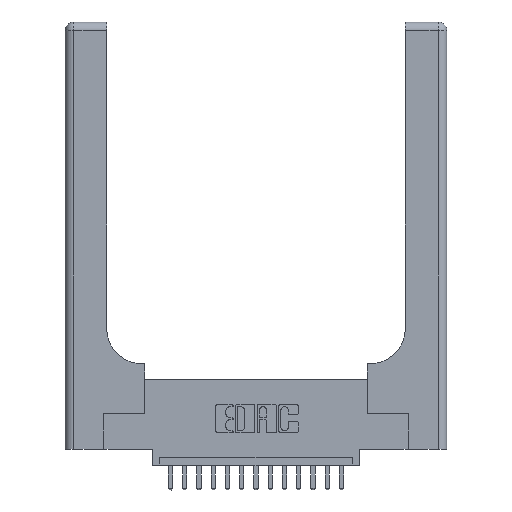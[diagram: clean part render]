
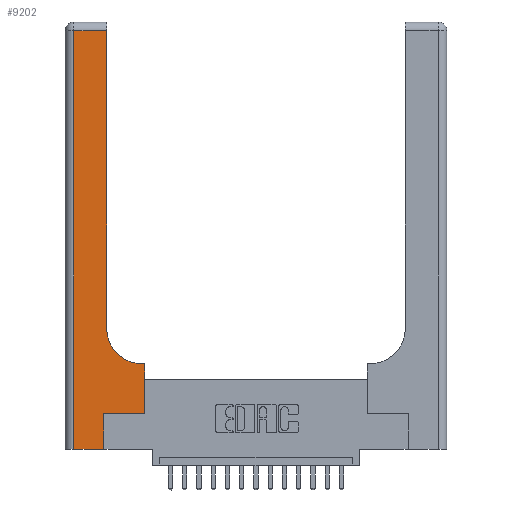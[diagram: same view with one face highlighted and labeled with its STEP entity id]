
A CAD part, top view. The second image highlights one B-rep face of the part: STEP entity #9202.
In plain terms, the highlighted planar face has unit normal (0, 0, 1).
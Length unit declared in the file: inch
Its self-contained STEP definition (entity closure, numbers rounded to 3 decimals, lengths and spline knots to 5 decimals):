
#174 = ORIENTED_EDGE ( 'NONE', *, *, #14792, .T. ) ;
#429 = AXIS2_PLACEMENT_3D ( 'NONE', #8814, #2917, #16340 ) ;
#547 = LINE ( 'NONE', #15109, #12341 ) ;
#780 = LINE ( 'NONE', #13860, #5628 ) ;
#890 = DIRECTION ( 'NONE',  ( -1., 0., 0. ) ) ;
#905 = VECTOR ( 'NONE', #5362, 39.37008 ) ;
#1137 = ORIENTED_EDGE ( 'NONE', *, *, #15764, .T. ) ;
#1366 = CARTESIAN_POINT ( 'NONE',  ( 0.5415, 0.6, 0.37 ) ) ;
#1576 = AXIS2_PLACEMENT_3D ( 'NONE', #3415, #16846, #8022 ) ;
#1577 = VERTEX_POINT ( 'NONE', #15545 ) ;
#1743 = ORIENTED_EDGE ( 'NONE', *, *, #8934, .T. ) ;
#1853 = DIRECTION ( 'NONE',  ( 0., -1., 0. ) ) ;
#2070 = CARTESIAN_POINT ( 'NONE',  ( 0.5585, 0.25, 0.37 ) ) ;
#2392 = ORIENTED_EDGE ( 'NONE', *, *, #12185, .T. ) ;
#2446 = VECTOR ( 'NONE', #13163, 39.37008 ) ;
#2524 = EDGE_CURVE ( 'NONE', #10962, #1577, #6870, .T. ) ;
#2917 = DIRECTION ( 'NONE',  ( 0., 0., -1. ) ) ;
#3000 = LINE ( 'NONE', #2070, #18255 ) ;
#3244 = VERTEX_POINT ( 'NONE', #11967 ) ;
#3305 = DIRECTION ( 'NONE',  ( 0., 1., 0. ) ) ;
#3332 = LINE ( 'NONE', #14197, #3804 ) ;
#3349 = LINE ( 'NONE', #17883, #9839 ) ;
#3415 = CARTESIAN_POINT ( 'NONE',  ( 0.5415, 0.85, 0.37 ) ) ;
#3541 = ORIENTED_EDGE ( 'NONE', *, *, #13657, .T. ) ;
#3584 = DIRECTION ( 'NONE',  ( -1., 0., 0. ) ) ;
#3741 = VERTEX_POINT ( 'NONE', #14222 ) ;
#3804 = VECTOR ( 'NONE', #890, 39.37008 ) ;
#4351 = ORIENTED_EDGE ( 'NONE', *, *, #8559, .T. ) ;
#4579 = VERTEX_POINT ( 'NONE', #15843 ) ;
#5362 = DIRECTION ( 'NONE',  ( 1., 0., 0. ) ) ;
#5628 = VECTOR ( 'NONE', #3584, 39.37008 ) ;
#5959 = PLANE ( 'NONE',  #429 ) ;
#6191 = EDGE_CURVE ( 'NONE', #10422, #10962, #10361, .T. ) ;
#6575 = DIRECTION ( 'NONE',  ( 1., 0., 0. ) ) ;
#6870 = LINE ( 'NONE', #7242, #2446 ) ;
#7242 = CARTESIAN_POINT ( 'NONE',  ( 0.269, 0., 0.37 ) ) ;
#7471 = FACE_OUTER_BOUND ( 'NONE', #10198, .T. ) ;
#8022 = DIRECTION ( 'NONE',  ( 1., 0., 0. ) ) ;
#8158 = EDGE_CURVE ( 'NONE', #3741, #10422, #3349, .T. ) ;
#8294 = VERTEX_POINT ( 'NONE', #16320 ) ;
#8559 = EDGE_CURVE ( 'NONE', #3244, #14511, #3332, .T. ) ;
#8814 = CARTESIAN_POINT ( 'NONE',  ( 0., 3., 0.37 ) ) ;
#8934 = EDGE_CURVE ( 'NONE', #4579, #3741, #780, .T. ) ;
#9202 = ADVANCED_FACE ( 'NONE', ( #7471 ), #5959, .F. ) ;
#9839 = VECTOR ( 'NONE', #1853, 39.37008 ) ;
#10198 = EDGE_LOOP ( 'NONE', ( #2392, #1743, #11842, #12910, #16523, #1137, #174, #4351, #3541 ) ) ;
#10361 = LINE ( 'NONE', #11030, #14723 ) ;
#10422 = VERTEX_POINT ( 'NONE', #16434 ) ;
#10962 = VERTEX_POINT ( 'NONE', #10972 ) ;
#10972 = CARTESIAN_POINT ( 'NONE',  ( 0.269, 0., 0.37 ) ) ;
#11030 = CARTESIAN_POINT ( 'NONE',  ( 0., 0., 0.37 ) ) ;
#11842 = ORIENTED_EDGE ( 'NONE', *, *, #8158, .T. ) ;
#11967 = CARTESIAN_POINT ( 'NONE',  ( 0.5585, 0.6, 0.37 ) ) ;
#12185 = EDGE_CURVE ( 'NONE', #8294, #4579, #547, .T. ) ;
#12341 = VECTOR ( 'NONE', #3305, 39.37008 ) ;
#12528 = VERTEX_POINT ( 'NONE', #14565 ) ;
#12698 = LINE ( 'NONE', #12970, #905 ) ;
#12910 = ORIENTED_EDGE ( 'NONE', *, *, #6191, .T. ) ;
#12970 = CARTESIAN_POINT ( 'NONE',  ( 0.269, 0.25, 0.37 ) ) ;
#13163 = DIRECTION ( 'NONE',  ( 0., 1., 0. ) ) ;
#13657 = EDGE_CURVE ( 'NONE', #14511, #8294, #15516, .T. ) ;
#13860 = CARTESIAN_POINT ( 'NONE',  ( 0., 2.94, 0.37 ) ) ;
#14197 = CARTESIAN_POINT ( 'NONE',  ( 0.2915, 0.6, 0.37 ) ) ;
#14222 = CARTESIAN_POINT ( 'NONE',  ( 0.06, 2.94, 0.37 ) ) ;
#14511 = VERTEX_POINT ( 'NONE', #1366 ) ;
#14565 = CARTESIAN_POINT ( 'NONE',  ( 0.5585, 0.25, 0.37 ) ) ;
#14723 = VECTOR ( 'NONE', #6575, 39.37008 ) ;
#14792 = EDGE_CURVE ( 'NONE', #12528, #3244, #3000, .T. ) ;
#15109 = CARTESIAN_POINT ( 'NONE',  ( 0.2915, 3., 0.37 ) ) ;
#15516 = CIRCLE ( 'NONE', #1576, 0.25 ) ;
#15545 = CARTESIAN_POINT ( 'NONE',  ( 0.269, 0.25, 0.37 ) ) ;
#15764 = EDGE_CURVE ( 'NONE', #1577, #12528, #12698, .T. ) ;
#15843 = CARTESIAN_POINT ( 'NONE',  ( 0.2915, 2.94, 0.37 ) ) ;
#16320 = CARTESIAN_POINT ( 'NONE',  ( 0.2915, 0.85, 0.37 ) ) ;
#16340 = DIRECTION ( 'NONE',  ( -1., 0., 0. ) ) ;
#16434 = CARTESIAN_POINT ( 'NONE',  ( 0.06, 0., 0.37 ) ) ;
#16523 = ORIENTED_EDGE ( 'NONE', *, *, #2524, .T. ) ;
#16846 = DIRECTION ( 'NONE',  ( 0., 0., -1. ) ) ;
#16870 = DIRECTION ( 'NONE',  ( 0., 1., 0. ) ) ;
#17883 = CARTESIAN_POINT ( 'NONE',  ( 0.06, 3., 0.37 ) ) ;
#18255 = VECTOR ( 'NONE', #16870, 39.37008 ) ;
